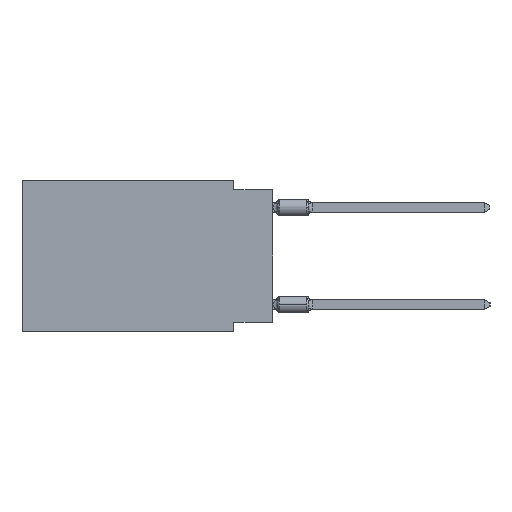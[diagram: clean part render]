
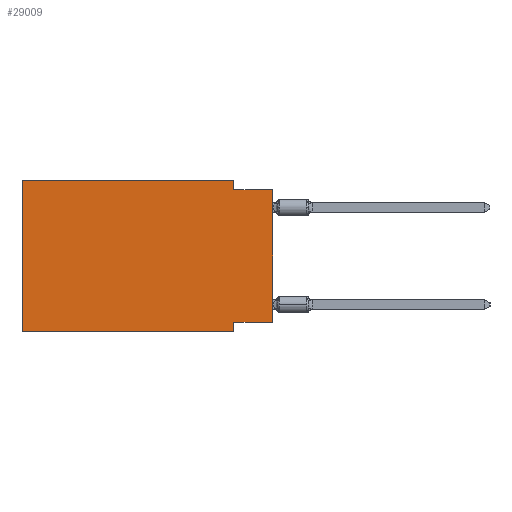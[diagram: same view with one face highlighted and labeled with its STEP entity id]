
A CAD part, left-side view. The second image highlights one B-rep face of the part: STEP entity #29009.
In plain terms, the highlighted planar face has unit normal (-1, 0, 0).
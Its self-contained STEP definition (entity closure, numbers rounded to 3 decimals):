
#141 = DIRECTION ( 'NONE',  ( 0., 0., -1. ) ) ;
#579 = CARTESIAN_POINT ( 'NONE',  ( 0., 2.54, 0. ) ) ;
#1288 = CARTESIAN_POINT ( 'NONE',  ( 0., 2.54, -0.635 ) ) ;
#2061 = VECTOR ( 'NONE', #23992, 1000. ) ;
#2217 = CARTESIAN_POINT ( 'NONE',  ( 0., 16.383, -9.906 ) ) ;
#2676 = DIRECTION ( 'NONE',  ( 0., -1., 0. ) ) ;
#3004 = EDGE_CURVE ( 'NONE', #7486, #15343, #19647, .T. ) ;
#3009 = CARTESIAN_POINT ( 'NONE',  ( 0., 0., -9.271 ) ) ;
#3085 = ORIENTED_EDGE ( 'NONE', *, *, #20040, .F. ) ;
#4144 = VERTEX_POINT ( 'NONE', #1288 ) ;
#4196 = CARTESIAN_POINT ( 'NONE',  ( 0., 16.383, 0. ) ) ;
#4874 = VECTOR ( 'NONE', #5873, 1000. ) ;
#5706 = LINE ( 'NONE', #27538, #30186 ) ;
#5873 = DIRECTION ( 'NONE',  ( 0., 1., 0. ) ) ;
#5989 = VERTEX_POINT ( 'NONE', #15480 ) ;
#6153 = CARTESIAN_POINT ( 'NONE',  ( 0., 2.54, -9.271 ) ) ;
#7349 = EDGE_CURVE ( 'NONE', #4144, #17762, #5706, .T. ) ;
#7486 = VERTEX_POINT ( 'NONE', #23027 ) ;
#7840 = VECTOR ( 'NONE', #7908, 1000. ) ;
#7861 = ORIENTED_EDGE ( 'NONE', *, *, #8332, .T. ) ;
#7908 = DIRECTION ( 'NONE',  ( 0., 0., -1. ) ) ;
#8076 = LINE ( 'NONE', #32777, #7840 ) ;
#8332 = EDGE_CURVE ( 'NONE', #7486, #17762, #14520, .T. ) ;
#8880 = VECTOR ( 'NONE', #12174, 1000. ) ;
#9363 = EDGE_CURVE ( 'NONE', #11466, #5989, #16340, .T. ) ;
#10574 = LINE ( 'NONE', #23617, #2061 ) ;
#10623 = VERTEX_POINT ( 'NONE', #12897 ) ;
#10888 = FACE_OUTER_BOUND ( 'NONE', #13317, .T. ) ;
#10972 = DIRECTION ( 'NONE',  ( 0., -1., 0. ) ) ;
#11051 = PLANE ( 'NONE',  #18421 ) ;
#11314 = EDGE_CURVE ( 'NONE', #11466, #10623, #23091, .T. ) ;
#11466 = VERTEX_POINT ( 'NONE', #16103 ) ;
#12174 = DIRECTION ( 'NONE',  ( 0., 0., 1. ) ) ;
#12249 = DIRECTION ( 'NONE',  ( 0., -1., 0. ) ) ;
#12897 = CARTESIAN_POINT ( 'NONE',  ( 0., 16.383, 0. ) ) ;
#13317 = EDGE_LOOP ( 'NONE', ( #7861, #15200, #3085, #31092, #15492, #21277, #29840, #18743 ) ) ;
#13732 = CARTESIAN_POINT ( 'NONE',  ( 0., 16.383, 0. ) ) ;
#14079 = VERTEX_POINT ( 'NONE', #579 ) ;
#14177 = VECTOR ( 'NONE', #17392, 1000. ) ;
#14520 = LINE ( 'NONE', #33535, #14177 ) ;
#15200 = ORIENTED_EDGE ( 'NONE', *, *, #7349, .F. ) ;
#15343 = VERTEX_POINT ( 'NONE', #6153 ) ;
#15480 = CARTESIAN_POINT ( 'NONE',  ( 0., 2.54, -9.906 ) ) ;
#15492 = ORIENTED_EDGE ( 'NONE', *, *, #11314, .F. ) ;
#16065 = DIRECTION ( 'NONE',  ( 1., 0., 0. ) ) ;
#16103 = CARTESIAN_POINT ( 'NONE',  ( 0., 16.383, -9.906 ) ) ;
#16340 = LINE ( 'NONE', #2217, #17578 ) ;
#17392 = DIRECTION ( 'NONE',  ( 0., 0., 1. ) ) ;
#17578 = VECTOR ( 'NONE', #10972, 1000. ) ;
#17762 = VERTEX_POINT ( 'NONE', #22657 ) ;
#18090 = CARTESIAN_POINT ( 'NONE',  ( 0., 16.383, 0. ) ) ;
#18421 = AXIS2_PLACEMENT_3D ( 'NONE', #13732, #16065, #141 ) ;
#18743 = ORIENTED_EDGE ( 'NONE', *, *, #3004, .F. ) ;
#19647 = LINE ( 'NONE', #3009, #4874 ) ;
#20040 = EDGE_CURVE ( 'NONE', #14079, #4144, #10574, .T. ) ;
#21277 = ORIENTED_EDGE ( 'NONE', *, *, #9363, .T. ) ;
#22657 = CARTESIAN_POINT ( 'NONE',  ( 0., 0., -0.635 ) ) ;
#23027 = CARTESIAN_POINT ( 'NONE',  ( 0., 0., -9.271 ) ) ;
#23091 = LINE ( 'NONE', #18090, #8880 ) ;
#23140 = EDGE_CURVE ( 'NONE', #15343, #5989, #8076, .T. ) ;
#23617 = CARTESIAN_POINT ( 'NONE',  ( 0., 2.54, 0. ) ) ;
#23992 = DIRECTION ( 'NONE',  ( 0., 0., -1. ) ) ;
#27538 = CARTESIAN_POINT ( 'NONE',  ( 0., 0., -0.635 ) ) ;
#29009 = ADVANCED_FACE ( 'NONE', ( #10888 ), #11051, .F. ) ;
#29840 = ORIENTED_EDGE ( 'NONE', *, *, #23140, .F. ) ;
#30186 = VECTOR ( 'NONE', #2676, 1000. ) ;
#31092 = ORIENTED_EDGE ( 'NONE', *, *, #32303, .F. ) ;
#31185 = VECTOR ( 'NONE', #12249, 1000. ) ;
#31602 = LINE ( 'NONE', #4196, #31185 ) ;
#32303 = EDGE_CURVE ( 'NONE', #10623, #14079, #31602, .T. ) ;
#32777 = CARTESIAN_POINT ( 'NONE',  ( 0., 2.54, -9.906 ) ) ;
#33535 = CARTESIAN_POINT ( 'NONE',  ( 0., 0., 0. ) ) ;
